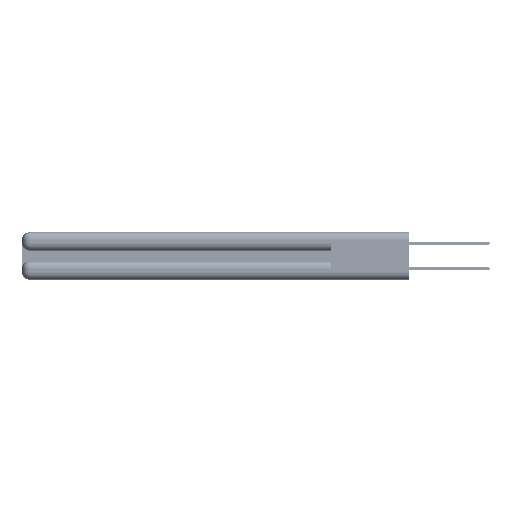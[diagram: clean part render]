
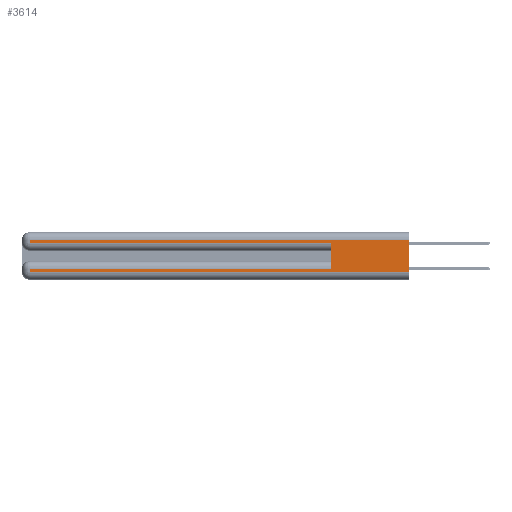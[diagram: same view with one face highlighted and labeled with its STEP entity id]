
A CAD part, left-side view. The second image highlights one B-rep face of the part: STEP entity #3614.
In plain terms, the highlighted planar face has unit normal (-1, 0, 0).
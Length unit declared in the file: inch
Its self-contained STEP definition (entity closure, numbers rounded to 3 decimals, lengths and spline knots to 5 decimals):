
#1512 = CARTESIAN_POINT ( 'NONE',  ( 0., 0., 0.06 ) ) ;
#2296 = VERTEX_POINT ( 'NONE', #46761 ) ;
#3614 = ADVANCED_FACE ( 'NONE', ( #12318 ), #33465, .F. ) ;
#4559 = EDGE_CURVE ( 'NONE', #25698, #30129, #8872, .T. ) ;
#4724 = CARTESIAN_POINT ( 'NONE',  ( 0., 2.94, 0.06 ) ) ;
#5554 = LINE ( 'NONE', #1512, #37147 ) ;
#5830 = VERTEX_POINT ( 'NONE', #49604 ) ;
#6952 = VECTOR ( 'NONE', #18184, 39.37008 ) ;
#7227 = CARTESIAN_POINT ( 'NONE',  ( 0., 2.94, 0.37 ) ) ;
#7904 = ORIENTED_EDGE ( 'NONE', *, *, #26607, .F. ) ;
#8237 = CARTESIAN_POINT ( 'NONE',  ( 0., 0., 0.37 ) ) ;
#8872 = LINE ( 'NONE', #50973, #52299 ) ;
#9606 = LINE ( 'NONE', #10269, #6952 ) ;
#10269 = CARTESIAN_POINT ( 'NONE',  ( 0., 2.94, 0.37 ) ) ;
#11117 = CARTESIAN_POINT ( 'NONE',  ( 0., 0.6, 0.145 ) ) ;
#11784 = CARTESIAN_POINT ( 'NONE',  ( 0., 2.94, 0.285 ) ) ;
#12221 = EDGE_CURVE ( 'NONE', #5830, #25698, #27461, .T. ) ;
#12318 = FACE_OUTER_BOUND ( 'NONE', #36250, .T. ) ;
#12475 = DIRECTION ( 'NONE',  ( 0., 0., -1. ) ) ;
#12720 = LINE ( 'NONE', #54372, #30502 ) ;
#13496 = ORIENTED_EDGE ( 'NONE', *, *, #4559, .T. ) ;
#14695 = DIRECTION ( 'NONE',  ( 0., -1., 0. ) ) ;
#15139 = LINE ( 'NONE', #8237, #49353 ) ;
#15520 = AXIS2_PLACEMENT_3D ( 'NONE', #42645, #17035, #16663 ) ;
#16663 = DIRECTION ( 'NONE',  ( 0., 0., -1. ) ) ;
#17012 = LINE ( 'NONE', #33103, #21595 ) ;
#17035 = DIRECTION ( 'NONE',  ( 1., 0., 0. ) ) ;
#17490 = LINE ( 'NONE', #11117, #22094 ) ;
#18184 = DIRECTION ( 'NONE',  ( 0., 0., -1. ) ) ;
#20119 = DIRECTION ( 'NONE',  ( 0., 0., -1. ) ) ;
#20303 = ORIENTED_EDGE ( 'NONE', *, *, #31476, .T. ) ;
#20871 = ORIENTED_EDGE ( 'NONE', *, *, #49108, .T. ) ;
#21595 = VECTOR ( 'NONE', #24113, 39.37008 ) ;
#22094 = VECTOR ( 'NONE', #32056, 39.37008 ) ;
#22621 = EDGE_CURVE ( 'NONE', #2296, #30129, #17490, .T. ) ;
#24113 = DIRECTION ( 'NONE',  ( 0., 1., 0. ) ) ;
#25698 = VERTEX_POINT ( 'NONE', #11784 ) ;
#26177 = VERTEX_POINT ( 'NONE', #39711 ) ;
#26607 = EDGE_CURVE ( 'NONE', #44896, #26177, #15139, .T. ) ;
#27461 = LINE ( 'NONE', #7227, #43948 ) ;
#27646 = CARTESIAN_POINT ( 'NONE',  ( 0., 0., 0.31 ) ) ;
#28093 = VERTEX_POINT ( 'NONE', #39366 ) ;
#29918 = VERTEX_POINT ( 'NONE', #4724 ) ;
#30129 = VERTEX_POINT ( 'NONE', #47766 ) ;
#30202 = ORIENTED_EDGE ( 'NONE', *, *, #12221, .T. ) ;
#30502 = VECTOR ( 'NONE', #39108, 39.37008 ) ;
#31476 = EDGE_CURVE ( 'NONE', #28093, #29918, #9606, .T. ) ;
#32056 = DIRECTION ( 'NONE',  ( 0., 0., 1. ) ) ;
#33103 = CARTESIAN_POINT ( 'NONE',  ( 0., 0., 0.085 ) ) ;
#33465 = PLANE ( 'NONE',  #15520 ) ;
#36250 = EDGE_LOOP ( 'NONE', ( #7904, #41585, #30202, #13496, #43947, #20871, #20303, #38588 ) ) ;
#37147 = VECTOR ( 'NONE', #14695, 39.37008 ) ;
#38588 = ORIENTED_EDGE ( 'NONE', *, *, #46029, .T. ) ;
#39108 = DIRECTION ( 'NONE',  ( 0., 1., 0. ) ) ;
#39366 = CARTESIAN_POINT ( 'NONE',  ( 0., 2.94, 0.085 ) ) ;
#39711 = CARTESIAN_POINT ( 'NONE',  ( 0., 0., 0.06 ) ) ;
#41585 = ORIENTED_EDGE ( 'NONE', *, *, #46515, .T. ) ;
#42645 = CARTESIAN_POINT ( 'NONE',  ( 0., 0., 0.37 ) ) ;
#43947 = ORIENTED_EDGE ( 'NONE', *, *, #22621, .F. ) ;
#43948 = VECTOR ( 'NONE', #20119, 39.37008 ) ;
#44896 = VERTEX_POINT ( 'NONE', #27646 ) ;
#46029 = EDGE_CURVE ( 'NONE', #29918, #26177, #5554, .T. ) ;
#46515 = EDGE_CURVE ( 'NONE', #44896, #5830, #12720, .T. ) ;
#46761 = CARTESIAN_POINT ( 'NONE',  ( 0., 0.6, 0.085 ) ) ;
#47766 = CARTESIAN_POINT ( 'NONE',  ( 0., 0.6, 0.285 ) ) ;
#48397 = DIRECTION ( 'NONE',  ( 0., -1., 0. ) ) ;
#49108 = EDGE_CURVE ( 'NONE', #2296, #28093, #17012, .T. ) ;
#49353 = VECTOR ( 'NONE', #12475, 39.37008 ) ;
#49604 = CARTESIAN_POINT ( 'NONE',  ( 0., 2.94, 0.31 ) ) ;
#50973 = CARTESIAN_POINT ( 'NONE',  ( 0., 0., 0.285 ) ) ;
#52299 = VECTOR ( 'NONE', #48397, 39.37008 ) ;
#54372 = CARTESIAN_POINT ( 'NONE',  ( 0., 0., 0.31 ) ) ;
